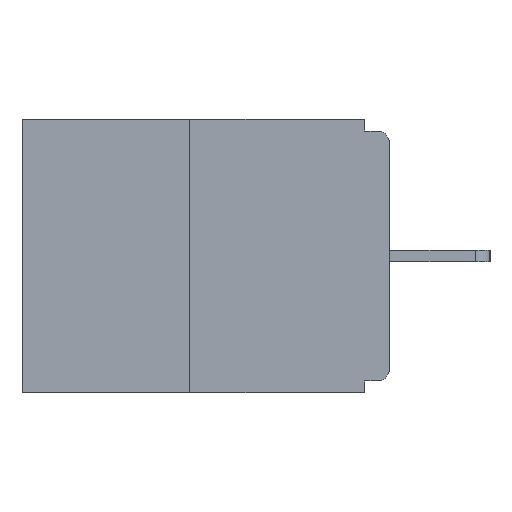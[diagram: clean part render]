
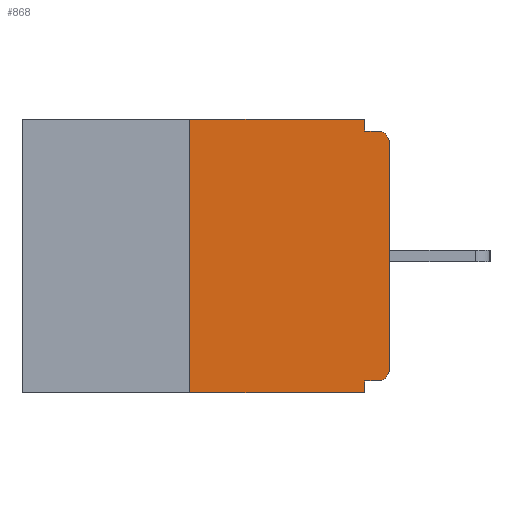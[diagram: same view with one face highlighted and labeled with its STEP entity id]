
A CAD part, left-side view. The second image highlights one B-rep face of the part: STEP entity #868.
In plain terms, the highlighted planar face has unit normal (-1, 0, 0).
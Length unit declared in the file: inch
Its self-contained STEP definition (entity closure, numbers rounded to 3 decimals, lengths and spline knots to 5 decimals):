
#78 = AXIS2_PLACEMENT_3D ( 'NONE', #17991, #15314, #15550 ) ;
#170 = LINE ( 'NONE', #755, #17709 ) ;
#697 = LINE ( 'NONE', #10747, #18715 ) ;
#755 = CARTESIAN_POINT ( 'NONE',  ( 0., 0.031, -0.343 ) ) ;
#829 = CARTESIAN_POINT ( 'NONE',  ( 0., 0.031, -0.015 ) ) ;
#868 = ADVANCED_FACE ( 'NONE', ( #9680 ), #19053, .F. ) ;
#874 = DIRECTION ( 'NONE',  ( 0., 0., 1. ) ) ;
#1131 = CARTESIAN_POINT ( 'NONE',  ( 0., 0.25, 0. ) ) ;
#2615 = CARTESIAN_POINT ( 'NONE',  ( 0., 0., 0. ) ) ;
#2750 = VECTOR ( 'NONE', #20685, 39.37008 ) ;
#3498 = CIRCLE ( 'NONE', #19569, 0.015 ) ;
#3621 = VECTOR ( 'NONE', #11231, 39.37008 ) ;
#3830 = LINE ( 'NONE', #18292, #7913 ) ;
#3834 = DIRECTION ( 'NONE',  ( 0., 0., -1. ) ) ;
#4011 = VERTEX_POINT ( 'NONE', #21267 ) ;
#4064 = AXIS2_PLACEMENT_3D ( 'NONE', #4490, #16291, #6246 ) ;
#4177 = ORIENTED_EDGE ( 'NONE', *, *, #7801, .F. ) ;
#4225 = DIRECTION ( 'NONE',  ( 0., -1., 0. ) ) ;
#4490 = CARTESIAN_POINT ( 'NONE',  ( 0., 0.015, -0.03 ) ) ;
#4896 = CARTESIAN_POINT ( 'NONE',  ( 0., 0., -0.03 ) ) ;
#5453 = CARTESIAN_POINT ( 'NONE',  ( 0., 0.015, -0.328 ) ) ;
#5472 = CARTESIAN_POINT ( 'NONE',  ( 0., 0., -0.313 ) ) ;
#5922 = VECTOR ( 'NONE', #874, 39.37008 ) ;
#6114 = EDGE_CURVE ( 'NONE', #10196, #11316, #3830, .T. ) ;
#6246 = DIRECTION ( 'NONE',  ( 0., 0., -1. ) ) ;
#6323 = EDGE_LOOP ( 'NONE', ( #13473, #4177, #18168, #20226, #16861, #15595, #16374, #15089, #20268, #21038 ) ) ;
#6456 = LINE ( 'NONE', #2615, #5922 ) ;
#7420 = VERTEX_POINT ( 'NONE', #9232 ) ;
#7586 = VECTOR ( 'NONE', #4225, 39.37008 ) ;
#7745 = CARTESIAN_POINT ( 'NONE',  ( 0., 0.031, 0. ) ) ;
#7801 = EDGE_CURVE ( 'NONE', #16513, #10196, #17388, .T. ) ;
#7913 = VECTOR ( 'NONE', #19562, 39.37008 ) ;
#8687 = EDGE_CURVE ( 'NONE', #13686, #4011, #21484, .T. ) ;
#9232 = CARTESIAN_POINT ( 'NONE',  ( 0., 0.015, -0.015 ) ) ;
#9445 = CIRCLE ( 'NONE', #4064, 0.015 ) ;
#9680 = FACE_OUTER_BOUND ( 'NONE', #6323, .T. ) ;
#9998 = DIRECTION ( 'NONE',  ( -1., 0., 0. ) ) ;
#10196 = VERTEX_POINT ( 'NONE', #1131 ) ;
#10747 = CARTESIAN_POINT ( 'NONE',  ( 0., 0.031, 0. ) ) ;
#11231 = DIRECTION ( 'NONE',  ( 0., 1., 0. ) ) ;
#11316 = VERTEX_POINT ( 'NONE', #7745 ) ;
#11320 = CARTESIAN_POINT ( 'NONE',  ( 0., 0., -0.328 ) ) ;
#11330 = LINE ( 'NONE', #12423, #2750 ) ;
#11544 = LINE ( 'NONE', #16053, #7586 ) ;
#12423 = CARTESIAN_POINT ( 'NONE',  ( 0., 0., -0.015 ) ) ;
#12435 = VECTOR ( 'NONE', #20934, 39.37008 ) ;
#13473 = ORIENTED_EDGE ( 'NONE', *, *, #6114, .F. ) ;
#13686 = VERTEX_POINT ( 'NONE', #5453 ) ;
#14589 = CARTESIAN_POINT ( 'NONE',  ( 0., 0.25, -0.343 ) ) ;
#14913 = EDGE_CURVE ( 'NONE', #15067, #7420, #11330, .T. ) ;
#15067 = VERTEX_POINT ( 'NONE', #829 ) ;
#15089 = ORIENTED_EDGE ( 'NONE', *, *, #20250, .T. ) ;
#15314 = DIRECTION ( 'NONE',  ( 1., 0., 0. ) ) ;
#15550 = DIRECTION ( 'NONE',  ( 0., 0., -1. ) ) ;
#15595 = ORIENTED_EDGE ( 'NONE', *, *, #19713, .T. ) ;
#15953 = EDGE_CURVE ( 'NONE', #16513, #21421, #11544, .T. ) ;
#16053 = CARTESIAN_POINT ( 'NONE',  ( 0., 0.46, -0.343 ) ) ;
#16068 = DIRECTION ( 'NONE',  ( 0., 0., -1. ) ) ;
#16291 = DIRECTION ( 'NONE',  ( -1., 0., 0. ) ) ;
#16374 = ORIENTED_EDGE ( 'NONE', *, *, #21049, .T. ) ;
#16513 = VERTEX_POINT ( 'NONE', #14589 ) ;
#16861 = ORIENTED_EDGE ( 'NONE', *, *, #8687, .F. ) ;
#17029 = CARTESIAN_POINT ( 'NONE',  ( 0., 0.031, -0.343 ) ) ;
#17388 = LINE ( 'NONE', #20979, #12435 ) ;
#17515 = VERTEX_POINT ( 'NONE', #5472 ) ;
#17709 = VECTOR ( 'NONE', #16068, 39.37008 ) ;
#17991 = CARTESIAN_POINT ( 'NONE',  ( 0., 0.46, 0. ) ) ;
#18168 = ORIENTED_EDGE ( 'NONE', *, *, #15953, .T. ) ;
#18292 = CARTESIAN_POINT ( 'NONE',  ( 0., 0.46, 0. ) ) ;
#18400 = EDGE_CURVE ( 'NONE', #4011, #21421, #170, .T. ) ;
#18715 = VECTOR ( 'NONE', #3834, 39.37008 ) ;
#18788 = EDGE_CURVE ( 'NONE', #11316, #15067, #697, .T. ) ;
#19053 = PLANE ( 'NONE',  #78 ) ;
#19562 = DIRECTION ( 'NONE',  ( 0., -1., 0. ) ) ;
#19569 = AXIS2_PLACEMENT_3D ( 'NONE', #19910, #9998, #21549 ) ;
#19713 = EDGE_CURVE ( 'NONE', #13686, #17515, #3498, .T. ) ;
#19753 = VERTEX_POINT ( 'NONE', #4896 ) ;
#19910 = CARTESIAN_POINT ( 'NONE',  ( 0., 0.015, -0.313 ) ) ;
#20226 = ORIENTED_EDGE ( 'NONE', *, *, #18400, .F. ) ;
#20250 = EDGE_CURVE ( 'NONE', #19753, #7420, #9445, .T. ) ;
#20268 = ORIENTED_EDGE ( 'NONE', *, *, #14913, .F. ) ;
#20685 = DIRECTION ( 'NONE',  ( 0., -1., 0. ) ) ;
#20934 = DIRECTION ( 'NONE',  ( 0., 0., 1. ) ) ;
#20979 = CARTESIAN_POINT ( 'NONE',  ( 0., 0.25, 0. ) ) ;
#21038 = ORIENTED_EDGE ( 'NONE', *, *, #18788, .F. ) ;
#21049 = EDGE_CURVE ( 'NONE', #17515, #19753, #6456, .T. ) ;
#21267 = CARTESIAN_POINT ( 'NONE',  ( 0., 0.031, -0.328 ) ) ;
#21421 = VERTEX_POINT ( 'NONE', #17029 ) ;
#21484 = LINE ( 'NONE', #11320, #3621 ) ;
#21549 = DIRECTION ( 'NONE',  ( 0., 0., -1. ) ) ;
